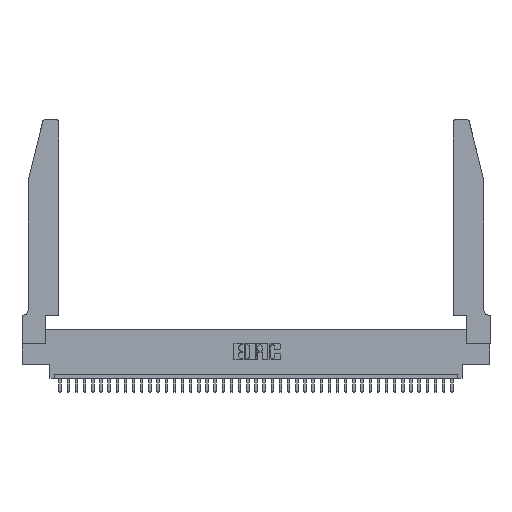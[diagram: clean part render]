
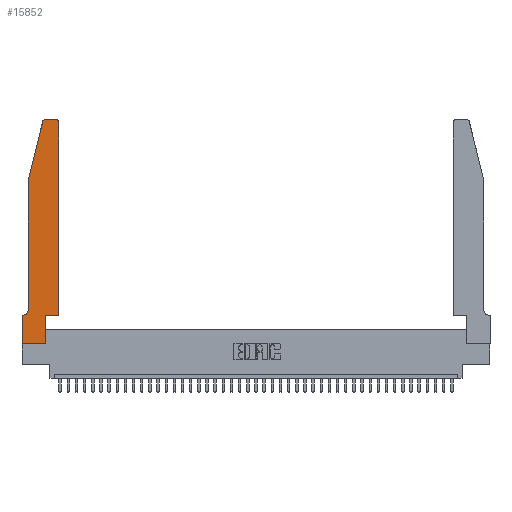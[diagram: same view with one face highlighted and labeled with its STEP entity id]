
A CAD part, top view. The second image highlights one B-rep face of the part: STEP entity #15852.
In plain terms, the highlighted planar face has unit normal (0, 0, 1).
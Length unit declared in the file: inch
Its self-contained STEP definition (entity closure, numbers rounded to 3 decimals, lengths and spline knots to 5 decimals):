
#103 = ORIENTED_EDGE ( 'NONE', *, *, #32561, .T. ) ;
#528 = EDGE_CURVE ( 'NONE', #21783, #36358, #29071, .T. ) ;
#792 = ORIENTED_EDGE ( 'NONE', *, *, #1012, .T. ) ;
#1012 = EDGE_CURVE ( 'NONE', #13217, #20864, #24120, .T. ) ;
#1587 = CARTESIAN_POINT ( 'NONE',  ( 0.0055, 0.42, 0.37 ) ) ;
#1621 = DIRECTION ( 'NONE',  ( -1., 0., 0. ) ) ;
#1641 = CARTESIAN_POINT ( 'NONE',  ( 0.4505, 0.35, 0.37 ) ) ;
#1781 = DIRECTION ( 'NONE',  ( 1., 0., 0. ) ) ;
#2046 = EDGE_CURVE ( 'NONE', #32816, #21783, #33332, .T. ) ;
#2051 = ORIENTED_EDGE ( 'NONE', *, *, #34970, .T. ) ;
#2534 = CARTESIAN_POINT ( 'NONE',  ( 0.2865, 0.35, 0.37 ) ) ;
#2778 = AXIS2_PLACEMENT_3D ( 'NONE', #24572, #9957, #10231 ) ;
#3141 = CIRCLE ( 'NONE', #7863, 0.03 ) ;
#3366 = CARTESIAN_POINT ( 'NONE',  ( 0.4505, 0.35, 0.37 ) ) ;
#4113 = VECTOR ( 'NONE', #20302, 39.37008 ) ;
#4561 = VERTEX_POINT ( 'NONE', #24923 ) ;
#4605 = DIRECTION ( 'NONE',  ( 0., -1., 0. ) ) ;
#5072 = CARTESIAN_POINT ( 'NONE',  ( 0.4505, 0.35, 0.37 ) ) ;
#5120 = VERTEX_POINT ( 'NONE', #3366 ) ;
#5892 = EDGE_CURVE ( 'NONE', #20864, #25964, #34950, .T. ) ;
#6638 = CARTESIAN_POINT ( 'NONE',  ( 0.0055, 0.35, 0.37 ) ) ;
#6852 = ORIENTED_EDGE ( 'NONE', *, *, #32329, .T. ) ;
#7005 = VERTEX_POINT ( 'NONE', #40906 ) ;
#7863 = AXIS2_PLACEMENT_3D ( 'NONE', #28417, #37379, #9449 ) ;
#8645 = CARTESIAN_POINT ( 'NONE',  ( 0.4505, 2.72, 0.37 ) ) ;
#8843 = CARTESIAN_POINT ( 'NONE',  ( 0.25487, 2.72718, 0.37 ) ) ;
#9449 = DIRECTION ( 'NONE',  ( 1., 0., 0. ) ) ;
#9957 = DIRECTION ( 'NONE',  ( 0., 0., 1. ) ) ;
#10023 = ORIENTED_EDGE ( 'NONE', *, *, #5892, .T. ) ;
#10138 = CIRCLE ( 'NONE', #20326, 0.03 ) ;
#10231 = DIRECTION ( 'NONE',  ( 1., 0., 0. ) ) ;
#10831 = CARTESIAN_POINT ( 'NONE',  ( 0.0755, 2., 0.37 ) ) ;
#11115 = VECTOR ( 'NONE', #1781, 39.37008 ) ;
#11216 = CARTESIAN_POINT ( 'NONE',  ( 0.284, 2.72, 0.37 ) ) ;
#11673 = CARTESIAN_POINT ( 'NONE',  ( 0.2605, 2.75, 0.37 ) ) ;
#12050 = LINE ( 'NONE', #11673, #37276 ) ;
#13217 = VERTEX_POINT ( 'NONE', #26923 ) ;
#14127 = DIRECTION ( 'NONE',  ( 0., 0., 1. ) ) ;
#14384 = DIRECTION ( 'NONE',  ( 0., 0., -1. ) ) ;
#14438 = DIRECTION ( 'NONE',  ( 0., 1., 0. ) ) ;
#15243 = VECTOR ( 'NONE', #34727, 39.37008 ) ;
#15510 = ORIENTED_EDGE ( 'NONE', *, *, #24062, .T. ) ;
#15852 = ADVANCED_FACE ( 'NONE', ( #28637 ), #37511, .T. ) ;
#16855 = AXIS2_PLACEMENT_3D ( 'NONE', #1587, #14384, #17612 ) ;
#17375 = DIRECTION ( 'NONE',  ( 1., 0., 0. ) ) ;
#17557 = CARTESIAN_POINT ( 'NONE',  ( 0.0755, 2., 0.37 ) ) ;
#17612 = DIRECTION ( 'NONE',  ( -1., 0., 0. ) ) ;
#18244 = VECTOR ( 'NONE', #35291, 39.37008 ) ;
#18351 = CARTESIAN_POINT ( 'NONE',  ( 0.2865, 0., 0.37 ) ) ;
#18697 = EDGE_CURVE ( 'NONE', #4561, #35859, #10138, .T. ) ;
#19530 = CARTESIAN_POINT ( 'NONE',  ( 0.0755, 2., 0.37 ) ) ;
#20080 = LINE ( 'NONE', #19530, #33869 ) ;
#20302 = DIRECTION ( 'NONE',  ( 0., -1., 0. ) ) ;
#20326 = AXIS2_PLACEMENT_3D ( 'NONE', #11216, #14127, #17375 ) ;
#20864 = VERTEX_POINT ( 'NONE', #18351 ) ;
#21586 = CARTESIAN_POINT ( 'NONE',  ( 0.0755, 0.35, 0.37 ) ) ;
#21634 = CARTESIAN_POINT ( 'NONE',  ( 0.2865, 0.35, 0.37 ) ) ;
#21754 = LINE ( 'NONE', #5072, #26472 ) ;
#21783 = VERTEX_POINT ( 'NONE', #6638 ) ;
#22865 = VERTEX_POINT ( 'NONE', #8645 ) ;
#24062 = EDGE_CURVE ( 'NONE', #5120, #22865, #21754, .T. ) ;
#24120 = LINE ( 'NONE', #26958, #32453 ) ;
#24572 = CARTESIAN_POINT ( 'NONE',  ( 0., 0.35, 0.37 ) ) ;
#24923 = CARTESIAN_POINT ( 'NONE',  ( 0.284, 2.75, 0.37 ) ) ;
#25111 = EDGE_LOOP ( 'NONE', ( #37242, #27035, #34694, #6852, #25350, #27239, #2051, #792, #10023, #37977, #15510, #103 ) ) ;
#25350 = ORIENTED_EDGE ( 'NONE', *, *, #2046, .T. ) ;
#25964 = VERTEX_POINT ( 'NONE', #21634 ) ;
#26385 = LINE ( 'NONE', #10831, #4113 ) ;
#26472 = VECTOR ( 'NONE', #14438, 39.37008 ) ;
#26923 = CARTESIAN_POINT ( 'NONE',  ( 0., 0., 0.37 ) ) ;
#26958 = CARTESIAN_POINT ( 'NONE',  ( 0., 0., 0.37 ) ) ;
#27035 = ORIENTED_EDGE ( 'NONE', *, *, #18697, .T. ) ;
#27148 = VECTOR ( 'NONE', #4605, 39.37008 ) ;
#27239 = ORIENTED_EDGE ( 'NONE', *, *, #528, .T. ) ;
#27359 = CARTESIAN_POINT ( 'NONE',  ( 0., 0.35, 0.37 ) ) ;
#27907 = EDGE_CURVE ( 'NONE', #35859, #35636, #20080, .T. ) ;
#28417 = CARTESIAN_POINT ( 'NONE',  ( 0.4205, 2.72, 0.37 ) ) ;
#28637 = FACE_OUTER_BOUND ( 'NONE', #25111, .T. ) ;
#28778 = EDGE_CURVE ( 'NONE', #7005, #4561, #12050, .T. ) ;
#29071 = LINE ( 'NONE', #21586, #15243 ) ;
#31665 = DIRECTION ( 'NONE',  ( -0.239, -0.971, 0. ) ) ;
#32329 = EDGE_CURVE ( 'NONE', #35636, #32816, #26385, .T. ) ;
#32453 = VECTOR ( 'NONE', #33806, 39.37008 ) ;
#32561 = EDGE_CURVE ( 'NONE', #22865, #7005, #3141, .T. ) ;
#32816 = VERTEX_POINT ( 'NONE', #35766 ) ;
#33332 = CIRCLE ( 'NONE', #16855, 0.07 ) ;
#33806 = DIRECTION ( 'NONE',  ( 1., 0., 0. ) ) ;
#33869 = VECTOR ( 'NONE', #31665, 39.37008 ) ;
#34694 = ORIENTED_EDGE ( 'NONE', *, *, #27907, .T. ) ;
#34727 = DIRECTION ( 'NONE',  ( -1., 0., 0. ) ) ;
#34950 = LINE ( 'NONE', #2534, #18244 ) ;
#34970 = EDGE_CURVE ( 'NONE', #36358, #13217, #37496, .T. ) ;
#35291 = DIRECTION ( 'NONE',  ( 0., 1., 0. ) ) ;
#35636 = VERTEX_POINT ( 'NONE', #17557 ) ;
#35766 = CARTESIAN_POINT ( 'NONE',  ( 0.0755, 0.42, 0.37 ) ) ;
#35859 = VERTEX_POINT ( 'NONE', #8843 ) ;
#36358 = VERTEX_POINT ( 'NONE', #27359 ) ;
#37242 = ORIENTED_EDGE ( 'NONE', *, *, #28778, .T. ) ;
#37276 = VECTOR ( 'NONE', #1621, 39.37008 ) ;
#37379 = DIRECTION ( 'NONE',  ( 0., 0., 1. ) ) ;
#37496 = LINE ( 'NONE', #39135, #27148 ) ;
#37511 = PLANE ( 'NONE',  #2778 ) ;
#37552 = EDGE_CURVE ( 'NONE', #25964, #5120, #40823, .T. ) ;
#37977 = ORIENTED_EDGE ( 'NONE', *, *, #37552, .T. ) ;
#39135 = CARTESIAN_POINT ( 'NONE',  ( 0., 0., 0.37 ) ) ;
#40823 = LINE ( 'NONE', #1641, #11115 ) ;
#40906 = CARTESIAN_POINT ( 'NONE',  ( 0.4205, 2.75, 0.37 ) ) ;
